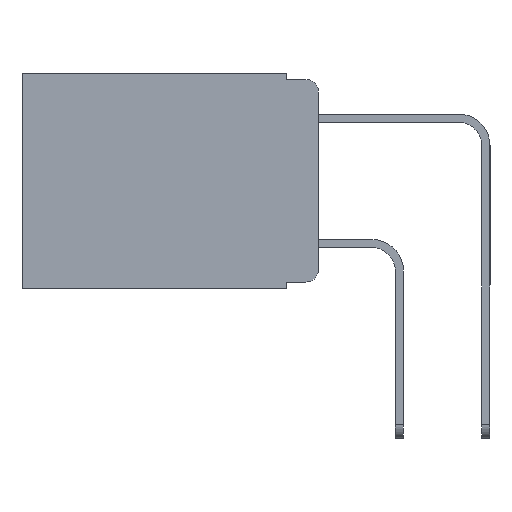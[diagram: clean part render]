
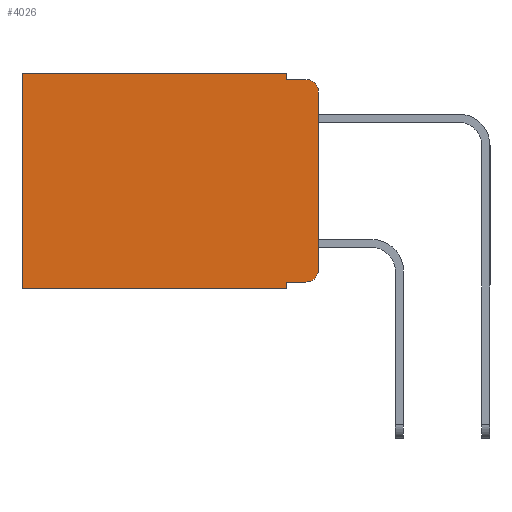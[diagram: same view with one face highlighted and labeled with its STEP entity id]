
A CAD part, left-side view. The second image highlights one B-rep face of the part: STEP entity #4026.
In plain terms, the highlighted planar face has unit normal (-1, 0, 0).
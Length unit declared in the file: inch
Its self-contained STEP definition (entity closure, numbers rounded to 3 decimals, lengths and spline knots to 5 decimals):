
#56 = VERTEX_POINT ( 'NONE', #13270 ) ;
#345 = ORIENTED_EDGE ( 'NONE', *, *, #13616, .F. ) ;
#368 = DIRECTION ( 'NONE',  ( 0., 0., -1. ) ) ;
#500 = DIRECTION ( 'NONE',  ( 0., 0., -1. ) ) ;
#535 = ORIENTED_EDGE ( 'NONE', *, *, #9282, .F. ) ;
#714 = ORIENTED_EDGE ( 'NONE', *, *, #7728, .T. ) ;
#766 = ORIENTED_EDGE ( 'NONE', *, *, #5437, .F. ) ;
#1247 = ORIENTED_EDGE ( 'NONE', *, *, #9080, .T. ) ;
#1342 = CARTESIAN_POINT ( 'NONE',  ( 0.298, 0., 0. ) ) ;
#1509 = LINE ( 'NONE', #10153, #12690 ) ;
#1546 = LINE ( 'NONE', #11885, #4544 ) ;
#1642 = DIRECTION ( 'NONE',  ( -1., 0., 0. ) ) ;
#1822 = VERTEX_POINT ( 'NONE', #2533 ) ;
#2118 = CARTESIAN_POINT ( 'NONE',  ( 0.298, 0., 0. ) ) ;
#2423 = EDGE_CURVE ( 'NONE', #7337, #10168, #12318, .T. ) ;
#2533 = CARTESIAN_POINT ( 'NONE',  ( 0.298, 0.473, 0. ) ) ;
#2931 = ORIENTED_EDGE ( 'NONE', *, *, #3158, .T. ) ;
#2968 = AXIS2_PLACEMENT_3D ( 'NONE', #5727, #4854, #4676 ) ;
#3001 = VERTEX_POINT ( 'NONE', #7934 ) ;
#3158 = EDGE_CURVE ( 'NONE', #3001, #7337, #5148, .T. ) ;
#3195 = CARTESIAN_POINT ( 'NONE',  ( 0.298, 0.02, -0.01 ) ) ;
#3468 = CARTESIAN_POINT ( 'NONE',  ( 0.298, 0.473, -0.343 ) ) ;
#3488 = CARTESIAN_POINT ( 'NONE',  ( 0.298, 0., -0.313 ) ) ;
#3794 = VECTOR ( 'NONE', #10376, 39.37008 ) ;
#4026 = ADVANCED_FACE ( 'NONE', ( #11784 ), #9032, .F. ) ;
#4335 = CARTESIAN_POINT ( 'NONE',  ( 0.298, 0.051, -0.01 ) ) ;
#4544 = VECTOR ( 'NONE', #13977, 39.37008 ) ;
#4673 = LINE ( 'NONE', #8472, #7677 ) ;
#4676 = DIRECTION ( 'NONE',  ( 0., 0., -1. ) ) ;
#4854 = DIRECTION ( 'NONE',  ( 1., 0., 0. ) ) ;
#5085 = VECTOR ( 'NONE', #368, 39.37008 ) ;
#5121 = VERTEX_POINT ( 'NONE', #9786 ) ;
#5148 = LINE ( 'NONE', #12884, #10774 ) ;
#5342 = DIRECTION ( 'NONE',  ( -1., 0., 0. ) ) ;
#5360 = CARTESIAN_POINT ( 'NONE',  ( 0.298, 0.02, -0.313 ) ) ;
#5377 = EDGE_CURVE ( 'NONE', #56, #10168, #11398, .T. ) ;
#5437 = EDGE_CURVE ( 'NONE', #3001, #5121, #11045, .T. ) ;
#5445 = DIRECTION ( 'NONE',  ( 0., -1., 0. ) ) ;
#5727 = CARTESIAN_POINT ( 'NONE',  ( 0.298, 0., 0. ) ) ;
#6217 = DIRECTION ( 'NONE',  ( 0., 0., -1. ) ) ;
#6408 = ORIENTED_EDGE ( 'NONE', *, *, #9764, .T. ) ;
#6592 = CIRCLE ( 'NONE', #6667, 0.02 ) ;
#6667 = AXIS2_PLACEMENT_3D ( 'NONE', #8406, #1642, #9572 ) ;
#7065 = VERTEX_POINT ( 'NONE', #3195 ) ;
#7337 = VERTEX_POINT ( 'NONE', #10402 ) ;
#7385 = VECTOR ( 'NONE', #11399, 39.37008 ) ;
#7677 = VECTOR ( 'NONE', #500, 39.37008 ) ;
#7711 = AXIS2_PLACEMENT_3D ( 'NONE', #5360, #5342, #6217 ) ;
#7728 = EDGE_CURVE ( 'NONE', #1822, #9013, #1509, .T. ) ;
#7934 = CARTESIAN_POINT ( 'NONE',  ( 0.298, 0.051, -0.333 ) ) ;
#7983 = ORIENTED_EDGE ( 'NONE', *, *, #5377, .F. ) ;
#8149 = LINE ( 'NONE', #4335, #10738 ) ;
#8275 = ORIENTED_EDGE ( 'NONE', *, *, #11459, .F. ) ;
#8406 = CARTESIAN_POINT ( 'NONE',  ( 0.298, 0.02, -0.03 ) ) ;
#8472 = CARTESIAN_POINT ( 'NONE',  ( 0.298, 0.051, 0. ) ) ;
#9013 = VERTEX_POINT ( 'NONE', #3468 ) ;
#9032 = PLANE ( 'NONE',  #2968 ) ;
#9061 = DIRECTION ( 'NONE',  ( 0., 0., -1. ) ) ;
#9080 = EDGE_CURVE ( 'NONE', #13701, #1822, #12680, .T. ) ;
#9280 = ORIENTED_EDGE ( 'NONE', *, *, #2423, .T. ) ;
#9282 = EDGE_CURVE ( 'NONE', #13701, #10398, #4673, .T. ) ;
#9572 = DIRECTION ( 'NONE',  ( 0., 0., -1. ) ) ;
#9644 = CARTESIAN_POINT ( 'NONE',  ( 0.298, 0.051, -0.01 ) ) ;
#9764 = EDGE_CURVE ( 'NONE', #56, #7065, #6592, .T. ) ;
#9786 = CARTESIAN_POINT ( 'NONE',  ( 0.298, 0.051, -0.343 ) ) ;
#10153 = CARTESIAN_POINT ( 'NONE',  ( 0.298, 0.473, 0. ) ) ;
#10168 = VERTEX_POINT ( 'NONE', #3488 ) ;
#10376 = DIRECTION ( 'NONE',  ( 0., 1., 0. ) ) ;
#10398 = VERTEX_POINT ( 'NONE', #9644 ) ;
#10402 = CARTESIAN_POINT ( 'NONE',  ( 0.298, 0.02, -0.333 ) ) ;
#10530 = CARTESIAN_POINT ( 'NONE',  ( 0.298, 0.051, 0. ) ) ;
#10738 = VECTOR ( 'NONE', #5445, 39.37008 ) ;
#10774 = VECTOR ( 'NONE', #11560, 39.37008 ) ;
#10972 = CARTESIAN_POINT ( 'NONE',  ( 0.298, 0.051, 0. ) ) ;
#11045 = LINE ( 'NONE', #10530, #7385 ) ;
#11398 = LINE ( 'NONE', #2118, #5085 ) ;
#11399 = DIRECTION ( 'NONE',  ( 0., 0., -1. ) ) ;
#11459 = EDGE_CURVE ( 'NONE', #10398, #7065, #8149, .T. ) ;
#11560 = DIRECTION ( 'NONE',  ( 0., -1., 0. ) ) ;
#11641 = EDGE_LOOP ( 'NONE', ( #7983, #6408, #8275, #535, #1247, #714, #345, #766, #2931, #9280 ) ) ;
#11784 = FACE_OUTER_BOUND ( 'NONE', #11641, .T. ) ;
#11885 = CARTESIAN_POINT ( 'NONE',  ( 0.298, 0., -0.343 ) ) ;
#12318 = CIRCLE ( 'NONE', #7711, 0.02 ) ;
#12680 = LINE ( 'NONE', #1342, #3794 ) ;
#12690 = VECTOR ( 'NONE', #9061, 39.37008 ) ;
#12884 = CARTESIAN_POINT ( 'NONE',  ( 0.298, 0.051, -0.333 ) ) ;
#13270 = CARTESIAN_POINT ( 'NONE',  ( 0.298, 0., -0.03 ) ) ;
#13616 = EDGE_CURVE ( 'NONE', #5121, #9013, #1546, .T. ) ;
#13701 = VERTEX_POINT ( 'NONE', #10972 ) ;
#13977 = DIRECTION ( 'NONE',  ( 0., 1., 0. ) ) ;
